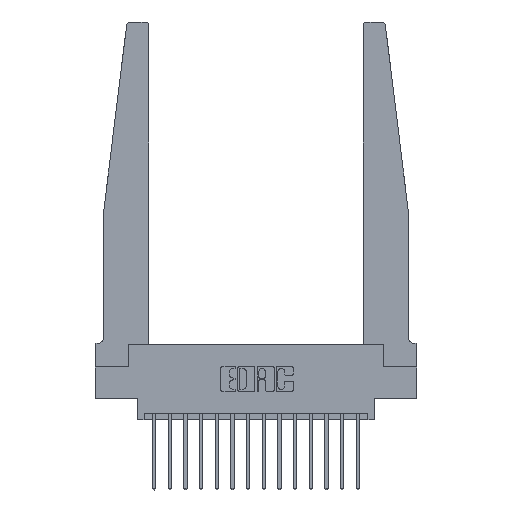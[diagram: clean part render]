
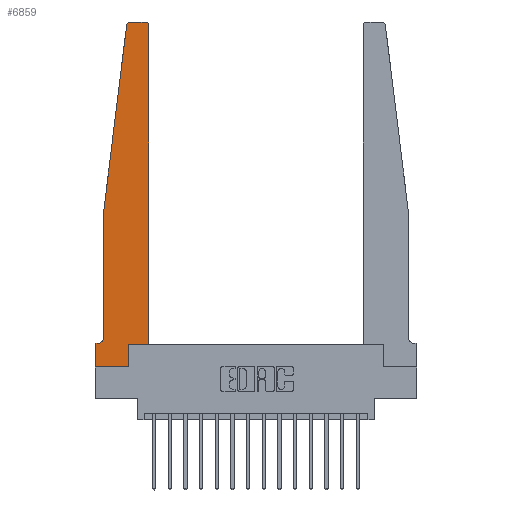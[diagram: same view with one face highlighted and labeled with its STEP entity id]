
A CAD part, top view. The second image highlights one B-rep face of the part: STEP entity #6859.
In plain terms, the highlighted planar face has unit normal (0, 0, 1).
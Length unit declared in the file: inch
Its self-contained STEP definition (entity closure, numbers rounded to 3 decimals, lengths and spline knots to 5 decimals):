
#228 = DIRECTION ( 'NONE',  ( 0., 0., 1. ) ) ;
#318 = DIRECTION ( 'NONE',  ( 0., 0., 1. ) ) ;
#599 = EDGE_CURVE ( 'NONE', #13094, #13233, #4200, .T. ) ;
#1065 = ORIENTED_EDGE ( 'NONE', *, *, #12298, .T. ) ;
#1302 = CARTESIAN_POINT ( 'NONE',  ( 0.425, 0.18, 0.37 ) ) ;
#1439 = CARTESIAN_POINT ( 'NONE',  ( 0.27653, 2.75, 0.37 ) ) ;
#1542 = LINE ( 'NONE', #15798, #8443 ) ;
#1597 = VECTOR ( 'NONE', #6038, 39.37008 ) ;
#1648 = AXIS2_PLACEMENT_3D ( 'NONE', #14470, #6224, #15858 ) ;
#1742 = LINE ( 'NONE', #1302, #8656 ) ;
#1785 = CIRCLE ( 'NONE', #1648, 0.05 ) ;
#1926 = AXIS2_PLACEMENT_3D ( 'NONE', #4308, #228, #9858 ) ;
#1932 = VERTEX_POINT ( 'NONE', #11393 ) ;
#2139 = DIRECTION ( 'NONE',  ( -1., 0., 0. ) ) ;
#2180 = LINE ( 'NONE', #2238, #9072 ) ;
#2190 = CARTESIAN_POINT ( 'NONE',  ( 0.425, 2.72, 0.37 ) ) ;
#2215 = LINE ( 'NONE', #12867, #16005 ) ;
#2238 = CARTESIAN_POINT ( 'NONE',  ( 0., 0., 0.37 ) ) ;
#2285 = VERTEX_POINT ( 'NONE', #6540 ) ;
#2401 = CARTESIAN_POINT ( 'NONE',  ( 0.065, 0.1875, 0.37 ) ) ;
#2655 = CIRCLE ( 'NONE', #4445, 0.03 ) ;
#2728 = EDGE_CURVE ( 'NONE', #16008, #14173, #1542, .T. ) ;
#2776 = VERTEX_POINT ( 'NONE', #3456 ) ;
#3183 = EDGE_CURVE ( 'NONE', #14173, #4392, #2215, .T. ) ;
#3213 = VECTOR ( 'NONE', #2139, 39.37008 ) ;
#3456 = CARTESIAN_POINT ( 'NONE',  ( 0., 0., 0.37 ) ) ;
#3591 = EDGE_LOOP ( 'NONE', ( #17206, #12830, #6185, #7097, #17004, #13767, #12855, #11665, #1065, #14715, #10005, #5435 ) ) ;
#3670 = VECTOR ( 'NONE', #5007, 39.37008 ) ;
#3706 = FACE_OUTER_BOUND ( 'NONE', #3591, .T. ) ;
#4200 = LINE ( 'NONE', #2401, #11071 ) ;
#4223 = EDGE_CURVE ( 'NONE', #2776, #6400, #2180, .T. ) ;
#4308 = CARTESIAN_POINT ( 'NONE',  ( 0., 0.1875, 0.37 ) ) ;
#4392 = VERTEX_POINT ( 'NONE', #15231 ) ;
#4445 = AXIS2_PLACEMENT_3D ( 'NONE', #8558, #318, #9928 ) ;
#4647 = CARTESIAN_POINT ( 'NONE',  ( 0.2605, 0.18, 0.37 ) ) ;
#5007 = DIRECTION ( 'NONE',  ( 0., 1., 0. ) ) ;
#5327 = EDGE_CURVE ( 'NONE', #1932, #12661, #6879, .T. ) ;
#5435 = ORIENTED_EDGE ( 'NONE', *, *, #14279, .T. ) ;
#5478 = CIRCLE ( 'NONE', #8235, 0.03 ) ;
#6038 = DIRECTION ( 'NONE',  ( 0., 1., 0. ) ) ;
#6185 = ORIENTED_EDGE ( 'NONE', *, *, #2728, .T. ) ;
#6188 = EDGE_CURVE ( 'NONE', #12661, #16008, #2655, .T. ) ;
#6224 = DIRECTION ( 'NONE',  ( 0., 0., -1. ) ) ;
#6264 = CARTESIAN_POINT ( 'NONE',  ( 0.2605, 0., 0.37 ) ) ;
#6400 = VERTEX_POINT ( 'NONE', #6264 ) ;
#6540 = CARTESIAN_POINT ( 'NONE',  ( 0.425, 0.18, 0.37 ) ) ;
#6859 = ADVANCED_FACE ( 'NONE', ( #3706 ), #8482, .T. ) ;
#6866 = CARTESIAN_POINT ( 'NONE',  ( 0., 0., 0.37 ) ) ;
#6879 = LINE ( 'NONE', #11761, #3213 ) ;
#6884 = DIRECTION ( 'NONE',  ( 0., 0., 1. ) ) ;
#7097 = ORIENTED_EDGE ( 'NONE', *, *, #3183, .T. ) ;
#8235 = AXIS2_PLACEMENT_3D ( 'NONE', #15130, #6884, #16523 ) ;
#8443 = VECTOR ( 'NONE', #10288, 39.37008 ) ;
#8482 = PLANE ( 'NONE',  #1926 ) ;
#8558 = CARTESIAN_POINT ( 'NONE',  ( 0.27653, 2.72, 0.37 ) ) ;
#8586 = EDGE_CURVE ( 'NONE', #13233, #2776, #13780, .T. ) ;
#8656 = VECTOR ( 'NONE', #12332, 39.37008 ) ;
#9072 = VECTOR ( 'NONE', #10509, 39.37008 ) ;
#9173 = CARTESIAN_POINT ( 'NONE',  ( 0.425, 0.18, 0.37 ) ) ;
#9858 = DIRECTION ( 'NONE',  ( 1., 0., 0. ) ) ;
#9928 = DIRECTION ( 'NONE',  ( 1., 0., 0. ) ) ;
#10005 = ORIENTED_EDGE ( 'NONE', *, *, #17598, .T. ) ;
#10115 = VECTOR ( 'NONE', #15108, 39.37008 ) ;
#10288 = DIRECTION ( 'NONE',  ( -0.122, -0.992, 0. ) ) ;
#10509 = DIRECTION ( 'NONE',  ( 1., 0., 0. ) ) ;
#10619 = CARTESIAN_POINT ( 'NONE',  ( 0.2605, 0.18, 0.37 ) ) ;
#10810 = CARTESIAN_POINT ( 'NONE',  ( 0.015, 0.1875, 0.37 ) ) ;
#11038 = CARTESIAN_POINT ( 'NONE',  ( 0., 0.1875, 0.37 ) ) ;
#11071 = VECTOR ( 'NONE', #14598, 39.37008 ) ;
#11393 = CARTESIAN_POINT ( 'NONE',  ( 0.395, 2.75, 0.37 ) ) ;
#11627 = VERTEX_POINT ( 'NONE', #2190 ) ;
#11665 = ORIENTED_EDGE ( 'NONE', *, *, #4223, .T. ) ;
#11761 = CARTESIAN_POINT ( 'NONE',  ( 0.25, 2.75, 0.37 ) ) ;
#11784 = CARTESIAN_POINT ( 'NONE',  ( 0.24675, 2.72367, 0.37 ) ) ;
#12298 = EDGE_CURVE ( 'NONE', #6400, #13561, #12592, .T. ) ;
#12332 = DIRECTION ( 'NONE',  ( 1., 0., 0. ) ) ;
#12592 = LINE ( 'NONE', #4647, #1597 ) ;
#12661 = VERTEX_POINT ( 'NONE', #1439 ) ;
#12830 = ORIENTED_EDGE ( 'NONE', *, *, #6188, .T. ) ;
#12855 = ORIENTED_EDGE ( 'NONE', *, *, #8586, .T. ) ;
#12867 = CARTESIAN_POINT ( 'NONE',  ( 0.065, 1.25, 0.37 ) ) ;
#13094 = VERTEX_POINT ( 'NONE', #10810 ) ;
#13233 = VERTEX_POINT ( 'NONE', #11038 ) ;
#13503 = CARTESIAN_POINT ( 'NONE',  ( 0.065, 1.25, 0.37 ) ) ;
#13561 = VERTEX_POINT ( 'NONE', #10619 ) ;
#13767 = ORIENTED_EDGE ( 'NONE', *, *, #599, .T. ) ;
#13780 = LINE ( 'NONE', #6866, #10115 ) ;
#14173 = VERTEX_POINT ( 'NONE', #13503 ) ;
#14279 = EDGE_CURVE ( 'NONE', #11627, #1932, #5478, .T. ) ;
#14470 = CARTESIAN_POINT ( 'NONE',  ( 0.015, 0.2375, 0.37 ) ) ;
#14598 = DIRECTION ( 'NONE',  ( -1., 0., 0. ) ) ;
#14661 = LINE ( 'NONE', #9173, #3670 ) ;
#14715 = ORIENTED_EDGE ( 'NONE', *, *, #16302, .T. ) ;
#15108 = DIRECTION ( 'NONE',  ( 0., -1., 0. ) ) ;
#15130 = CARTESIAN_POINT ( 'NONE',  ( 0.395, 2.72, 0.37 ) ) ;
#15231 = CARTESIAN_POINT ( 'NONE',  ( 0.065, 0.2375, 0.37 ) ) ;
#15307 = EDGE_CURVE ( 'NONE', #4392, #13094, #1785, .T. ) ;
#15798 = CARTESIAN_POINT ( 'NONE',  ( 0.065, 1.25, 0.37 ) ) ;
#15858 = DIRECTION ( 'NONE',  ( -1., 0., 0. ) ) ;
#16005 = VECTOR ( 'NONE', #17035, 39.37008 ) ;
#16008 = VERTEX_POINT ( 'NONE', #11784 ) ;
#16302 = EDGE_CURVE ( 'NONE', #13561, #2285, #1742, .T. ) ;
#16523 = DIRECTION ( 'NONE',  ( 1., 0., 0. ) ) ;
#17004 = ORIENTED_EDGE ( 'NONE', *, *, #15307, .T. ) ;
#17035 = DIRECTION ( 'NONE',  ( 0., -1., 0. ) ) ;
#17206 = ORIENTED_EDGE ( 'NONE', *, *, #5327, .T. ) ;
#17598 = EDGE_CURVE ( 'NONE', #2285, #11627, #14661, .T. ) ;
